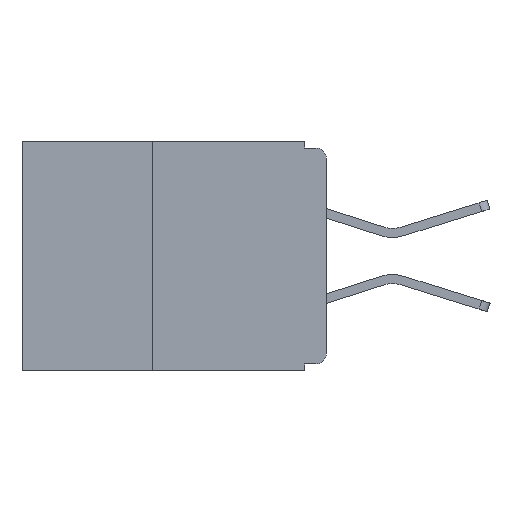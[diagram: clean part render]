
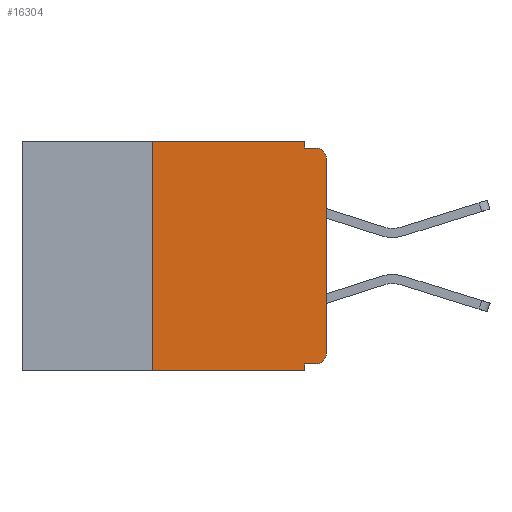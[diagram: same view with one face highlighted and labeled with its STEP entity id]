
A CAD part, left-side view. The second image highlights one B-rep face of the part: STEP entity #16304.
In plain terms, the highlighted planar face has unit normal (-1, 0, 0).
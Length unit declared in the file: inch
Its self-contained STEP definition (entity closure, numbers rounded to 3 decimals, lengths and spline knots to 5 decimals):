
#236 = VERTEX_POINT ( 'NONE', #1335 ) ;
#529 = CARTESIAN_POINT ( 'NONE',  ( 0., 0.437, 0. ) ) ;
#875 = DIRECTION ( 'NONE',  ( 0., 1., 0. ) ) ;
#1222 = VERTEX_POINT ( 'NONE', #7228 ) ;
#1335 = CARTESIAN_POINT ( 'NONE',  ( 0., 0.031, -0.32 ) ) ;
#1726 = ORIENTED_EDGE ( 'NONE', *, *, #7643, .T. ) ;
#1747 = AXIS2_PLACEMENT_3D ( 'NONE', #529, #4700, #14319 ) ;
#1976 = LINE ( 'NONE', #5179, #5188 ) ;
#2394 = CIRCLE ( 'NONE', #16074, 0.015 ) ;
#2888 = CARTESIAN_POINT ( 'NONE',  ( 0., 0.437, -0.33 ) ) ;
#2980 = CARTESIAN_POINT ( 'NONE',  ( 0., 0.031, -0.01 ) ) ;
#3291 = EDGE_CURVE ( 'NONE', #15133, #15689, #4864, .T. ) ;
#3322 = PLANE ( 'NONE',  #1747 ) ;
#3499 = EDGE_CURVE ( 'NONE', #13520, #15133, #15160, .T. ) ;
#3607 = CARTESIAN_POINT ( 'NONE',  ( 0., 0.015, -0.025 ) ) ;
#3629 = EDGE_CURVE ( 'NONE', #15210, #13520, #6580, .T. ) ;
#3720 = DIRECTION ( 'NONE',  ( 0., -1., 0. ) ) ;
#3819 = CARTESIAN_POINT ( 'NONE',  ( 0., 0.437, 0. ) ) ;
#3905 = VERTEX_POINT ( 'NONE', #11038 ) ;
#4419 = VECTOR ( 'NONE', #14165, 39.37008 ) ;
#4484 = FACE_OUTER_BOUND ( 'NONE', #9639, .T. ) ;
#4486 = CIRCLE ( 'NONE', #14978, 0.015 ) ;
#4700 = DIRECTION ( 'NONE',  ( 1., 0., 0. ) ) ;
#4721 = ORIENTED_EDGE ( 'NONE', *, *, #4983, .F. ) ;
#4864 = LINE ( 'NONE', #14051, #4419 ) ;
#4958 = EDGE_CURVE ( 'NONE', #1222, #3905, #2394, .T. ) ;
#4983 = EDGE_CURVE ( 'NONE', #15689, #14475, #1976, .T. ) ;
#4996 = DIRECTION ( 'NONE',  ( 0., 0., -1. ) ) ;
#5071 = VECTOR ( 'NONE', #12173, 39.37008 ) ;
#5104 = CARTESIAN_POINT ( 'NONE',  ( 0., 0., 0. ) ) ;
#5179 = CARTESIAN_POINT ( 'NONE',  ( 0., 0., -0.01 ) ) ;
#5188 = VECTOR ( 'NONE', #9320, 39.37008 ) ;
#5200 = VERTEX_POINT ( 'NONE', #5692 ) ;
#5309 = CARTESIAN_POINT ( 'NONE',  ( 0., 0.031, -0.33 ) ) ;
#5592 = ORIENTED_EDGE ( 'NONE', *, *, #3291, .F. ) ;
#5692 = CARTESIAN_POINT ( 'NONE',  ( 0., 0.031, -0.33 ) ) ;
#5745 = LINE ( 'NONE', #2888, #8539 ) ;
#6222 = ORIENTED_EDGE ( 'NONE', *, *, #6796, .T. ) ;
#6559 = DIRECTION ( 'NONE',  ( -1., 0., 0. ) ) ;
#6580 = LINE ( 'NONE', #16013, #9368 ) ;
#6796 = EDGE_CURVE ( 'NONE', #7729, #14475, #4486, .T. ) ;
#7199 = CARTESIAN_POINT ( 'NONE',  ( 0., 0., -0.025 ) ) ;
#7228 = CARTESIAN_POINT ( 'NONE',  ( 0., 0.015, -0.32 ) ) ;
#7453 = LINE ( 'NONE', #5104, #14765 ) ;
#7643 = EDGE_CURVE ( 'NONE', #15210, #5200, #5745, .T. ) ;
#7729 = VERTEX_POINT ( 'NONE', #7199 ) ;
#8539 = VECTOR ( 'NONE', #13877, 39.37008 ) ;
#8706 = LINE ( 'NONE', #5309, #5071 ) ;
#8997 = CARTESIAN_POINT ( 'NONE',  ( 0., 0.25, 0. ) ) ;
#9122 = CARTESIAN_POINT ( 'NONE',  ( 0., 0., -0.32 ) ) ;
#9268 = ORIENTED_EDGE ( 'NONE', *, *, #4958, .T. ) ;
#9320 = DIRECTION ( 'NONE',  ( 0., -1., 0. ) ) ;
#9368 = VECTOR ( 'NONE', #15794, 39.37008 ) ;
#9395 = VECTOR ( 'NONE', #875, 39.37008 ) ;
#9639 = EDGE_LOOP ( 'NONE', ( #12681, #6222, #4721, #5592, #14620, #11422, #1726, #14419, #11643, #9268 ) ) ;
#10147 = CARTESIAN_POINT ( 'NONE',  ( 0., 0.25, -0.33 ) ) ;
#11038 = CARTESIAN_POINT ( 'NONE',  ( 0., 0., -0.305 ) ) ;
#11076 = CARTESIAN_POINT ( 'NONE',  ( 0., 0.015, -0.01 ) ) ;
#11309 = EDGE_CURVE ( 'NONE', #1222, #236, #16626, .T. ) ;
#11422 = ORIENTED_EDGE ( 'NONE', *, *, #3629, .F. ) ;
#11643 = ORIENTED_EDGE ( 'NONE', *, *, #11309, .F. ) ;
#11966 = VECTOR ( 'NONE', #3720, 39.37008 ) ;
#12045 = EDGE_CURVE ( 'NONE', #236, #5200, #8706, .T. ) ;
#12173 = DIRECTION ( 'NONE',  ( 0., 0., -1. ) ) ;
#12681 = ORIENTED_EDGE ( 'NONE', *, *, #17087, .T. ) ;
#12727 = CARTESIAN_POINT ( 'NONE',  ( 0., 0.031, 0. ) ) ;
#13224 = DIRECTION ( 'NONE',  ( -1., 0., 0. ) ) ;
#13520 = VERTEX_POINT ( 'NONE', #8997 ) ;
#13877 = DIRECTION ( 'NONE',  ( 0., -1., 0. ) ) ;
#14051 = CARTESIAN_POINT ( 'NONE',  ( 0., 0.031, 0. ) ) ;
#14165 = DIRECTION ( 'NONE',  ( 0., 0., -1. ) ) ;
#14319 = DIRECTION ( 'NONE',  ( 0., 0., -1. ) ) ;
#14419 = ORIENTED_EDGE ( 'NONE', *, *, #12045, .F. ) ;
#14475 = VERTEX_POINT ( 'NONE', #11076 ) ;
#14620 = ORIENTED_EDGE ( 'NONE', *, *, #3499, .F. ) ;
#14700 = DIRECTION ( 'NONE',  ( 0., 0., 1. ) ) ;
#14765 = VECTOR ( 'NONE', #14700, 39.37008 ) ;
#14771 = CARTESIAN_POINT ( 'NONE',  ( 0., 0.015, -0.305 ) ) ;
#14978 = AXIS2_PLACEMENT_3D ( 'NONE', #3607, #13224, #4996 ) ;
#15133 = VERTEX_POINT ( 'NONE', #12727 ) ;
#15160 = LINE ( 'NONE', #3819, #11966 ) ;
#15210 = VERTEX_POINT ( 'NONE', #10147 ) ;
#15689 = VERTEX_POINT ( 'NONE', #2980 ) ;
#15794 = DIRECTION ( 'NONE',  ( 0., 0., 1. ) ) ;
#16013 = CARTESIAN_POINT ( 'NONE',  ( 0., 0.25, -0.33 ) ) ;
#16074 = AXIS2_PLACEMENT_3D ( 'NONE', #14771, #6559, #16122 ) ;
#16122 = DIRECTION ( 'NONE',  ( 0., 0., -1. ) ) ;
#16304 = ADVANCED_FACE ( 'NONE', ( #4484 ), #3322, .F. ) ;
#16626 = LINE ( 'NONE', #9122, #9395 ) ;
#17087 = EDGE_CURVE ( 'NONE', #3905, #7729, #7453, .T. ) ;
